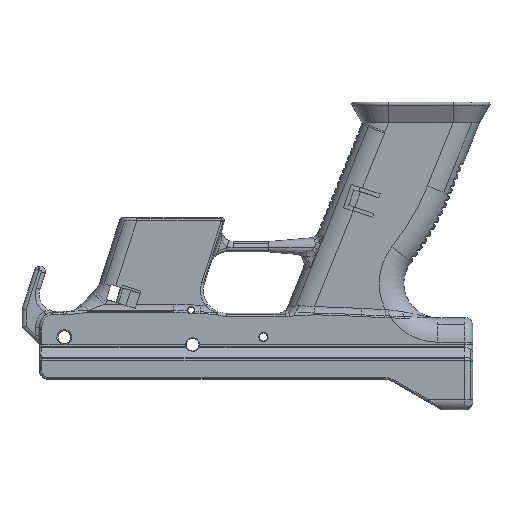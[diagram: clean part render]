
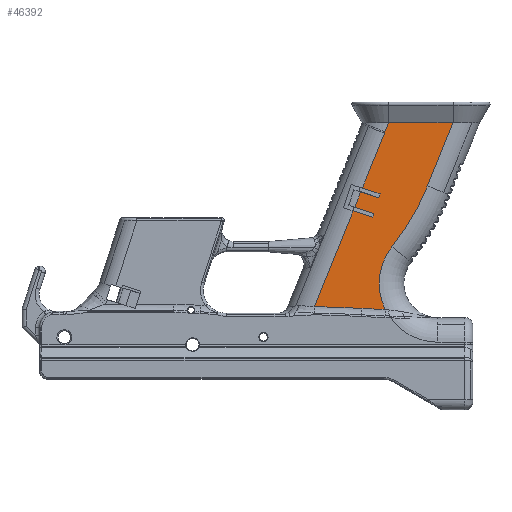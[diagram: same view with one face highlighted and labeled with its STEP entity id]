
A CAD part, front view. The second image highlights one B-rep face of the part: STEP entity #46392.
In plain terms, the highlighted planar face has unit normal (0, -1, 0).
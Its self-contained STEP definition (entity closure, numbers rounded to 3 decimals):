
#311 = CARTESIAN_POINT ( 'NONE',  ( 2.375, -14.625, 7.416 ) ) ;
#549 = CARTESIAN_POINT ( 'NONE',  ( 88.199, -14.625, 23.402 ) ) ;
#585 = DIRECTION ( 'NONE',  ( -0.305, 0., -0.952 ) ) ;
#586 = CARTESIAN_POINT ( 'NONE',  ( 76.954, -14.625, -62.561 ) ) ;
#992 = EDGE_CURVE ( 'NONE', #54169, #9474, #40982, .T. ) ;
#1714 = VERTEX_POINT ( 'NONE', #38137 ) ;
#2118 = ORIENTED_EDGE ( 'NONE', *, *, #14292, .F. ) ;
#2234 = DIRECTION ( 'NONE',  ( 0.992, 0., 0.126 ) ) ;
#2522 = EDGE_CURVE ( 'NONE', #8023, #25858, #39548, .T. ) ;
#2682 = DIRECTION ( 'NONE',  ( 0., 0., -1. ) ) ;
#2922 = CARTESIAN_POINT ( 'NONE',  ( 82.172, -14.625, -18.143 ) ) ;
#4147 = CARTESIAN_POINT ( 'NONE',  ( 91.6, -14.625, -32.517 ) ) ;
#4567 = CARTESIAN_POINT ( 'NONE',  ( 113.981, -14.625, -50.37 ) ) ;
#4719 = EDGE_CURVE ( 'NONE', #20407, #43985, #44143, .T. ) ;
#4798 = CIRCLE ( 'NONE', #43331, 17. ) ;
#5182 = LINE ( 'NONE', #34811, #31495 ) ;
#7678 = DIRECTION ( 'NONE',  ( 0.782, 0., -0.624 ) ) ;
#8023 = VERTEX_POINT ( 'NONE', #8868 ) ;
#8193 = CARTESIAN_POINT ( 'NONE',  ( 39.557, -14.625, -757.86 ) ) ;
#8806 = VECTOR ( 'NONE', #30924, 1000. ) ;
#8868 = CARTESIAN_POINT ( 'NONE',  ( 53.832, -14.625, -61.703 ) ) ;
#9474 = VERTEX_POINT ( 'NONE', #15466 ) ;
#9524 = CARTESIAN_POINT ( 'NONE',  ( 79.797, -14.625, -25.559 ) ) ;
#9961 = EDGE_CURVE ( 'NONE', #43985, #22553, #10737, .T. ) ;
#10004 = EDGE_CURVE ( 'NONE', #28500, #27932, #4798, .T. ) ;
#10737 = LINE ( 'NONE', #15404, #17087 ) ;
#11887 = DIRECTION ( 'NONE',  ( -0.375, 0., -0.927 ) ) ;
#12429 = LINE ( 'NONE', #32746, #38954 ) ;
#12563 = CARTESIAN_POINT ( 'NONE',  ( 85.832, -14.625, -6.715 ) ) ;
#13230 = ORIENTED_EDGE ( 'NONE', *, *, #992, .F. ) ;
#13370 = DIRECTION ( 'NONE',  ( 0., -1., 0. ) ) ;
#13554 = AXIS2_PLACEMENT_3D ( 'NONE', #8193, #53184, #20862 ) ;
#13620 = LINE ( 'NONE', #16935, #28359 ) ;
#13878 = DIRECTION ( 'NONE',  ( -0.952, 0., 0.305 ) ) ;
#14146 = CARTESIAN_POINT ( 'NONE',  ( 121.365, -14.625, 27.958 ) ) ;
#14292 = EDGE_CURVE ( 'NONE', #9474, #34351, #47681, .T. ) ;
#14795 = DIRECTION ( 'NONE',  ( 0.375, 0., 0.927 ) ) ;
#14833 = ORIENTED_EDGE ( 'NONE', *, *, #15699, .F. ) ;
#15042 = CARTESIAN_POINT ( 'NONE',  ( 69.665, -14.625, 27.958 ) ) ;
#15166 = CARTESIAN_POINT ( 'NONE',  ( 90.04, -14.625, 27.958 ) ) ;
#15404 = CARTESIAN_POINT ( 'NONE',  ( 88.226, -14.625, -9.581 ) ) ;
#15466 = CARTESIAN_POINT ( 'NONE',  ( 88.326, -14.625, -63.079 ) ) ;
#15486 = ORIENTED_EDGE ( 'NONE', *, *, #16247, .F. ) ;
#15568 = ORIENTED_EDGE ( 'NONE', *, *, #45575, .F. ) ;
#15699 = EDGE_CURVE ( 'NONE', #34351, #8023, #46822, .T. ) ;
#16247 = EDGE_CURVE ( 'NONE', #44920, #20407, #13620, .T. ) ;
#16333 = VERTEX_POINT ( 'NONE', #14146 ) ;
#16714 = EDGE_CURVE ( 'NONE', #1714, #54169, #26646, .T. ) ;
#16935 = CARTESIAN_POINT ( 'NONE',  ( 2.985, -14.625, 9.32 ) ) ;
#17015 = VERTEX_POINT ( 'NONE', #27119 ) ;
#17087 = VECTOR ( 'NONE', #31604, 1000. ) ;
#17097 = DIRECTION ( 'NONE',  ( -0.952, 0., 0.305 ) ) ;
#17824 = VERTEX_POINT ( 'NONE', #15166 ) ;
#17839 = ORIENTED_EDGE ( 'NONE', *, *, #46741, .T. ) ;
#18185 = DIRECTION ( 'NONE',  ( 0.375, 0., 0.927 ) ) ;
#18479 = VECTOR ( 'NONE', #42991, 1000. ) ;
#19770 = DIRECTION ( 'NONE',  ( 0.891, 0., -0.454 ) ) ;
#19983 = CARTESIAN_POINT ( 'NONE',  ( 70.22, -14.625, -21.141 ) ) ;
#20407 = VERTEX_POINT ( 'NONE', #21740 ) ;
#20862 = DIRECTION ( 'NONE',  ( -0.054, 0., -0.999 ) ) ;
#21168 = ORIENTED_EDGE ( 'NONE', *, *, #25508, .F. ) ;
#21503 = CARTESIAN_POINT ( 'NONE',  ( 82.782, -14.625, -16.238 ) ) ;
#21550 = ORIENTED_EDGE ( 'NONE', *, *, #4719, .F. ) ;
#21740 = CARTESIAN_POINT ( 'NONE',  ( 73.413, -14.625, -13.237 ) ) ;
#21761 = LINE ( 'NONE', #311, #36084 ) ;
#22553 = VERTEX_POINT ( 'NONE', #43887 ) ;
#22721 = LINE ( 'NONE', #39412, #18479 ) ;
#22777 = ORIENTED_EDGE ( 'NONE', *, *, #46657, .T. ) ;
#23000 = CARTESIAN_POINT ( 'NONE',  ( 76.418, -14.625, -5.799 ) ) ;
#23476 = VECTOR ( 'NONE', #14795, 1000. ) ;
#23580 = DIRECTION ( 'NONE',  ( 0., -1., 0. ) ) ;
#23683 = VECTOR ( 'NONE', #44395, 1000. ) ;
#23840 = VERTEX_POINT ( 'NONE', #2922 ) ;
#24340 = AXIS2_PLACEMENT_3D ( 'NONE', #4567, #13370, #7678 ) ;
#24682 = LINE ( 'NONE', #9524, #8806 ) ;
#25313 = ORIENTED_EDGE ( 'NONE', *, *, #34790, .T. ) ;
#25508 = EDGE_CURVE ( 'NONE', #17015, #28500, #35861, .T. ) ;
#25858 = VERTEX_POINT ( 'NONE', #37718 ) ;
#26646 = CIRCLE ( 'NONE', #45888, 118.894 ) ;
#27119 = CARTESIAN_POINT ( 'NONE',  ( 77.169, -14.625, -3.94 ) ) ;
#27507 = CARTESIAN_POINT ( 'NONE',  ( 72.175, -14.625, 29.078 ) ) ;
#27932 = VERTEX_POINT ( 'NONE', #549 ) ;
#28232 = CARTESIAN_POINT ( 'NONE',  ( 86.464, -14.625, -15.081 ) ) ;
#28359 = VECTOR ( 'NONE', #13878, 1000. ) ;
#28500 = VERTEX_POINT ( 'NONE', #41498 ) ;
#30711 = DIRECTION ( 'NONE',  ( 0.952, 0., -0.305 ) ) ;
#30924 = DIRECTION ( 'NONE',  ( -0.305, 0., -0.952 ) ) ;
#31255 = CARTESIAN_POINT ( 'NONE',  ( 70.22, -14.625, -21.141 ) ) ;
#31495 = VECTOR ( 'NONE', #30711, 1000. ) ;
#31504 = EDGE_LOOP ( 'NONE', ( #15486, #33474, #41619, #34804, #14833, #2118, #13230, #41485, #42638, #15568, #17839, #39044, #21168, #25313, #22777, #35135, #21550 ) ) ;
#31604 = DIRECTION ( 'NONE',  ( 0.952, 0., -0.305 ) ) ;
#31822 = DIRECTION ( 'NONE',  ( 0.037, 0., 0.999 ) ) ;
#32617 = PLANE ( 'NONE',  #52574 ) ;
#32746 = CARTESIAN_POINT ( 'NONE',  ( 111.761, -14.625, 4.188 ) ) ;
#33474 = ORIENTED_EDGE ( 'NONE', *, *, #39001, .T. ) ;
#33550 = LINE ( 'NONE', #38200, #52060 ) ;
#34351 = VERTEX_POINT ( 'NONE', #586 ) ;
#34529 = AXIS2_PLACEMENT_3D ( 'NONE', #52640, #40846, #31822 ) ;
#34790 = EDGE_CURVE ( 'NONE', #17015, #36215, #5182, .T. ) ;
#34804 = ORIENTED_EDGE ( 'NONE', *, *, #2522, .F. ) ;
#34811 = CARTESIAN_POINT ( 'NONE',  ( 88.836, -14.625, -7.677 ) ) ;
#35135 = ORIENTED_EDGE ( 'NONE', *, *, #9961, .F. ) ;
#35861 = LINE ( 'NONE', #19983, #48296 ) ;
#36084 = VECTOR ( 'NONE', #17097, 1000. ) ;
#36215 = VERTEX_POINT ( 'NONE', #12563 ) ;
#37718 = CARTESIAN_POINT ( 'NONE',  ( 72.662, -14.625, -15.097 ) ) ;
#38137 = CARTESIAN_POINT ( 'NONE',  ( 108.893, -14.625, -2.912 ) ) ;
#38200 = CARTESIAN_POINT ( 'NONE',  ( 79.797, -14.625, -25.559 ) ) ;
#38734 = EDGE_CURVE ( 'NONE', #16333, #1714, #12429, .T. ) ;
#38954 = VECTOR ( 'NONE', #11887, 1000. ) ;
#39001 = EDGE_CURVE ( 'NONE', #44920, #23840, #33550, .T. ) ;
#39044 = ORIENTED_EDGE ( 'NONE', *, *, #10004, .F. ) ;
#39412 = CARTESIAN_POINT ( 'NONE',  ( 106.929, -14.625, 69.761 ) ) ;
#39548 = LINE ( 'NONE', #43125, #41552 ) ;
#40283 = FACE_OUTER_BOUND ( 'NONE', #31504, .T. ) ;
#40846 = DIRECTION ( 'NONE',  ( 0., 1., 0. ) ) ;
#40982 = CIRCLE ( 'NONE', #24340, 28.63 ) ;
#41059 = DIRECTION ( 'NONE',  ( 0.375, 0., 0.927 ) ) ;
#41485 = ORIENTED_EDGE ( 'NONE', *, *, #16714, .F. ) ;
#41498 = CARTESIAN_POINT ( 'NONE',  ( 87.937, -14.625, 22.71 ) ) ;
#41552 = VECTOR ( 'NONE', #18185, 1000. ) ;
#41619 = ORIENTED_EDGE ( 'NONE', *, *, #52396, .T. ) ;
#42638 = ORIENTED_EDGE ( 'NONE', *, *, #38734, .F. ) ;
#42991 = DIRECTION ( 'NONE',  ( -0.375, 0., -0.927 ) ) ;
#43125 = CARTESIAN_POINT ( 'NONE',  ( 70.22, -14.625, -21.141 ) ) ;
#43331 = AXIS2_PLACEMENT_3D ( 'NONE', #27507, #44486, #2234 ) ;
#43887 = CARTESIAN_POINT ( 'NONE',  ( 85.222, -14.625, -8.619 ) ) ;
#43985 = VERTEX_POINT ( 'NONE', #23000 ) ;
#44143 = LINE ( 'NONE', #31255, #23476 ) ;
#44395 = DIRECTION ( 'NONE',  ( 1., 0., 0. ) ) ;
#44486 = DIRECTION ( 'NONE',  ( 0., -1., 0. ) ) ;
#44920 = VERTEX_POINT ( 'NONE', #21503 ) ;
#45575 = EDGE_CURVE ( 'NONE', #17824, #16333, #53428, .T. ) ;
#45888 = AXIS2_PLACEMENT_3D ( 'NONE', #48015, #52387, #19770 ) ;
#46392 = ADVANCED_FACE ( 'NONE', ( #40283 ), #32617, .T. ) ;
#46657 = EDGE_CURVE ( 'NONE', #36215, #22553, #24682, .T. ) ;
#46741 = EDGE_CURVE ( 'NONE', #17824, #27932, #22721, .T. ) ;
#46822 = CIRCLE ( 'NONE', #13554, 696.304 ) ;
#47681 = CIRCLE ( 'NONE', #34529, 689.416 ) ;
#48015 = CARTESIAN_POINT ( 'NONE',  ( -1.344, -14.625, 41.627 ) ) ;
#48296 = VECTOR ( 'NONE', #41059, 1000. ) ;
#52060 = VECTOR ( 'NONE', #585, 1000. ) ;
#52387 = DIRECTION ( 'NONE',  ( 0., 1., 0. ) ) ;
#52396 = EDGE_CURVE ( 'NONE', #23840, #25858, #21761, .T. ) ;
#52574 = AXIS2_PLACEMENT_3D ( 'NONE', #28232, #23580, #2682 ) ;
#52640 = CARTESIAN_POINT ( 'NONE',  ( 113.981, -14.625, 625.86 ) ) ;
#53184 = DIRECTION ( 'NONE',  ( 0., -1., 0. ) ) ;
#53428 = LINE ( 'NONE', #15042, #23683 ) ;
#54169 = VERTEX_POINT ( 'NONE', #4147 ) ;
